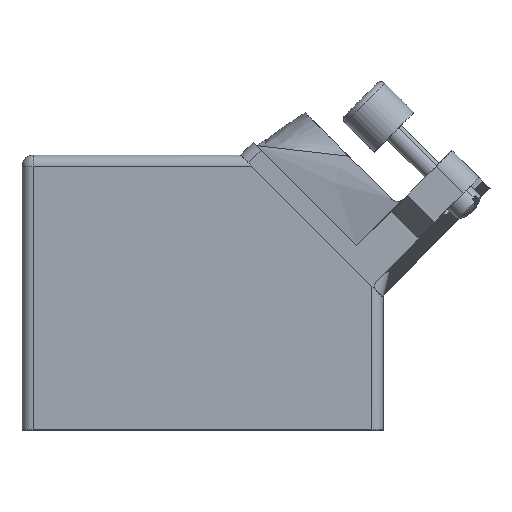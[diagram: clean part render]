
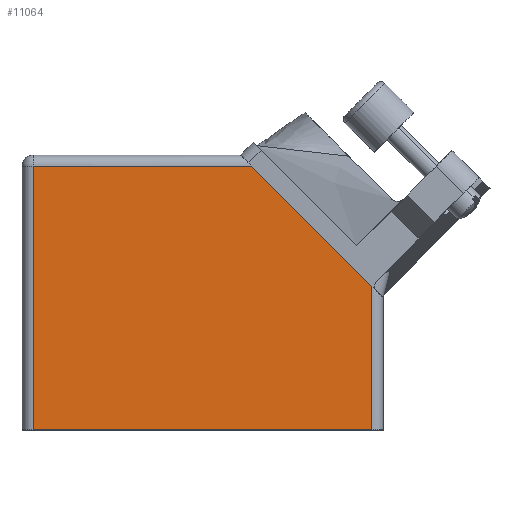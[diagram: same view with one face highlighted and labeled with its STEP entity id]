
A CAD part, top view. The second image highlights one B-rep face of the part: STEP entity #11064.
In plain terms, the highlighted planar face has unit normal (0, 0, 1).
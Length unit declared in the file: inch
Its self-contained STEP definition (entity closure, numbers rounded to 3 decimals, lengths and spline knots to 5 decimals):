
#425 = CARTESIAN_POINT ( 'NONE',  ( 0.062, 0., 0. ) ) ;
#499 = VERTEX_POINT ( 'NONE', #15435 ) ;
#631 = PLANE ( 'NONE',  #9929 ) ;
#925 = DIRECTION ( 'NONE',  ( 0., -1., 0. ) ) ;
#1953 = VECTOR ( 'NONE', #8170, 39.37008 ) ;
#2017 = DIRECTION ( 'NONE',  ( 1., 0., 0. ) ) ;
#2685 = EDGE_LOOP ( 'NONE', ( #13753, #12262, #2839, #14038, #2871 ) ) ;
#2839 = ORIENTED_EDGE ( 'NONE', *, *, #9969, .T. ) ;
#2871 = ORIENTED_EDGE ( 'NONE', *, *, #7167, .T. ) ;
#3003 = VECTOR ( 'NONE', #5074, 39.37008 ) ;
#3288 = LINE ( 'NONE', #5926, #1953 ) ;
#3951 = LINE ( 'NONE', #13737, #3003 ) ;
#4112 = VERTEX_POINT ( 'NONE', #6685 ) ;
#4173 = CARTESIAN_POINT ( 'NONE',  ( 0., 1.468, 0. ) ) ;
#4427 = FACE_OUTER_BOUND ( 'NONE', #2685, .T. ) ;
#4943 = VERTEX_POINT ( 'NONE', #425 ) ;
#5074 = DIRECTION ( 'NONE',  ( 1., 0., 0. ) ) ;
#5926 = CARTESIAN_POINT ( 'NONE',  ( 2.01, 0.737, 0. ) ) ;
#6024 = VERTEX_POINT ( 'NONE', #6934 ) ;
#6149 = CARTESIAN_POINT ( 'NONE',  ( 0.062, 0., 0. ) ) ;
#6685 = CARTESIAN_POINT ( 'NONE',  ( 1.948, 0., 0. ) ) ;
#6771 = DIRECTION ( 'NONE',  ( 0., 1., 0. ) ) ;
#6934 = CARTESIAN_POINT ( 'NONE',  ( 1.948, 0.799, 0. ) ) ;
#7167 = EDGE_CURVE ( 'NONE', #6024, #499, #3288, .T. ) ;
#7627 = VECTOR ( 'NONE', #6771, 39.37008 ) ;
#7997 = DIRECTION ( 'NONE',  ( -1., 0., 0. ) ) ;
#8170 = DIRECTION ( 'NONE',  ( -0.707, 0.707, 0. ) ) ;
#9766 = LINE ( 'NONE', #6149, #9843 ) ;
#9843 = VECTOR ( 'NONE', #925, 39.37008 ) ;
#9929 = AXIS2_PLACEMENT_3D ( 'NONE', #11576, #10439, #2017 ) ;
#9969 = EDGE_CURVE ( 'NONE', #4943, #4112, #3951, .T. ) ;
#10010 = LINE ( 'NONE', #12578, #7627 ) ;
#10327 = EDGE_CURVE ( 'NONE', #499, #10473, #11782, .T. ) ;
#10439 = DIRECTION ( 'NONE',  ( 0., 0., 1. ) ) ;
#10473 = VERTEX_POINT ( 'NONE', #14364 ) ;
#10934 = VECTOR ( 'NONE', #7997, 39.37008 ) ;
#11064 = ADVANCED_FACE ( 'NONE', ( #4427 ), #631, .T. ) ;
#11576 = CARTESIAN_POINT ( 'NONE',  ( 0., 0., 0. ) ) ;
#11782 = LINE ( 'NONE', #4173, #10934 ) ;
#11806 = EDGE_CURVE ( 'NONE', #4112, #6024, #10010, .T. ) ;
#12262 = ORIENTED_EDGE ( 'NONE', *, *, #12911, .T. ) ;
#12578 = CARTESIAN_POINT ( 'NONE',  ( 1.948, 0., 0. ) ) ;
#12911 = EDGE_CURVE ( 'NONE', #10473, #4943, #9766, .T. ) ;
#13737 = CARTESIAN_POINT ( 'NONE',  ( 0., 0., 0. ) ) ;
#13753 = ORIENTED_EDGE ( 'NONE', *, *, #10327, .T. ) ;
#14038 = ORIENTED_EDGE ( 'NONE', *, *, #11806, .T. ) ;
#14364 = CARTESIAN_POINT ( 'NONE',  ( 0.062, 1.468, 0. ) ) ;
#15435 = CARTESIAN_POINT ( 'NONE',  ( 1.279, 1.468, 0. ) ) ;
